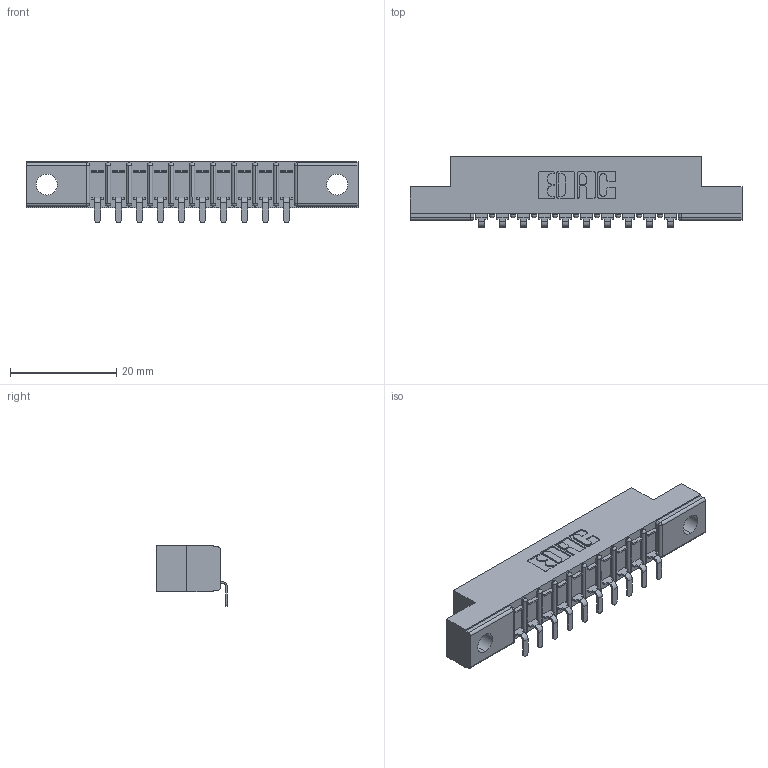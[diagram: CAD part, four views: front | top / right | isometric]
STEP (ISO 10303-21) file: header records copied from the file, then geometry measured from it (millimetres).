
FILE_DESCRIPTION (( 'STEP AP203' ), '1' );
FILE_NAME ('357-010-553-104.STEP', '2019-09-16T18:34:10', ( '' ), ( '' ), 'SwSTEP 2.0', 'SolidWorks 2016', '' );
FILE_SCHEMA (( 'CONFIG_CONTROL_DESIGN' ));
Length unit declared in the file: inch
Products named in the file (3): 307 Part_.156 Dia Mounting Holes; 307-290-002_553; 357-010-553-104
Assembly tree (11 placements, depth 2):
  357-010-553-104
    307 Part_.156 Dia Mounting Holes
    307-290-002_553  x10
Bounding box: 62.64 x 13.32 x 11.51 mm (x, y, z)
Volume: 4022.9 mm3; surface area: 6543.4 mm2
Topology: 11 solids, 11 shells, 923 faces, 2799 edges, 1834 vertices
Faces by surface type: plane 554, cylinder 347, sphere 22
Entity records: 13790 total; most frequent: CARTESIAN_POINT 2326, ORIENTED_EDGE 2314, DIRECTION 2267, EDGE_CURVE 1157, VECTOR 877, LINE 877, VERTEX_POINT 754, AXIS2_PLACEMENT_3D 695
